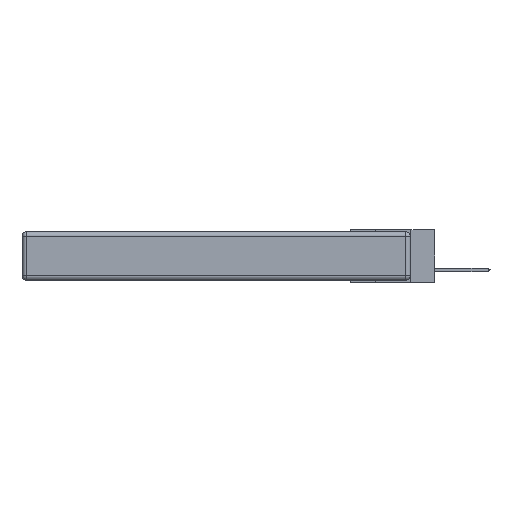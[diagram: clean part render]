
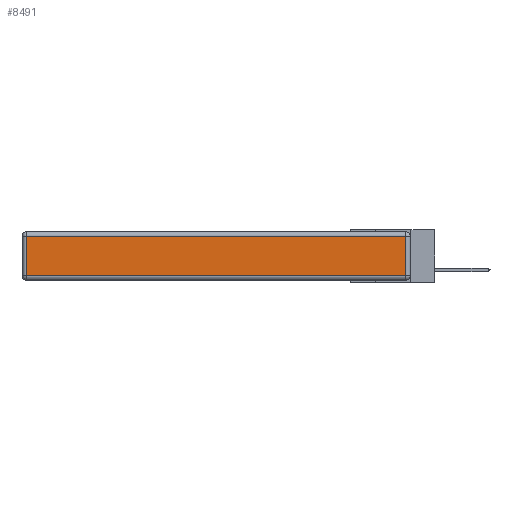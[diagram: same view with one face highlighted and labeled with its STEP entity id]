
A CAD part, left-side view. The second image highlights one B-rep face of the part: STEP entity #8491.
In plain terms, the highlighted planar face has unit normal (-1, 0, 0).
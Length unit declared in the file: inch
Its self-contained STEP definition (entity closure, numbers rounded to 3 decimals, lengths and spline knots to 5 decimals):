
#1834 = EDGE_CURVE ( 'NONE', #15540, #20115, #21368, .T. ) ;
#3686 = EDGE_CURVE ( 'NONE', #20085, #15540, #3948, .T. ) ;
#3948 = LINE ( 'NONE', #19818, #24108 ) ;
#4475 = VERTEX_POINT ( 'NONE', #6435 ) ;
#4882 = PLANE ( 'NONE',  #5160 ) ;
#5160 = AXIS2_PLACEMENT_3D ( 'NONE', #20413, #6901, #14629 ) ;
#6435 = CARTESIAN_POINT ( 'NONE',  ( 0., 2.72, -0.313 ) ) ;
#6901 = DIRECTION ( 'NONE',  ( -1., 0., 0. ) ) ;
#7764 = FACE_OUTER_BOUND ( 'NONE', #15975, .T. ) ;
#8491 = ADVANCED_FACE ( 'NONE', ( #7764 ), #4882, .T. ) ;
#8629 = LINE ( 'NONE', #18706, #10735 ) ;
#10615 = DIRECTION ( 'NONE',  ( 0., -1., 0. ) ) ;
#10735 = VECTOR ( 'NONE', #18450, 39.37008 ) ;
#10836 = ORIENTED_EDGE ( 'NONE', *, *, #1834, .T. ) ;
#10925 = EDGE_CURVE ( 'NONE', #20115, #4475, #8629, .T. ) ;
#11140 = ORIENTED_EDGE ( 'NONE', *, *, #17292, .T. ) ;
#12356 = VECTOR ( 'NONE', #18617, 39.37008 ) ;
#14629 = DIRECTION ( 'NONE',  ( 0., 0., 1. ) ) ;
#15354 = CARTESIAN_POINT ( 'NONE',  ( 0., 0.03, -0.313 ) ) ;
#15540 = VERTEX_POINT ( 'NONE', #19746 ) ;
#15975 = EDGE_LOOP ( 'NONE', ( #11140, #17421, #10836, #23685 ) ) ;
#17241 = VECTOR ( 'NONE', #10615, 39.37008 ) ;
#17292 = EDGE_CURVE ( 'NONE', #4475, #20085, #19646, .T. ) ;
#17421 = ORIENTED_EDGE ( 'NONE', *, *, #3686, .T. ) ;
#18450 = DIRECTION ( 'NONE',  ( 0., 0., -1. ) ) ;
#18617 = DIRECTION ( 'NONE',  ( 0., 1., 0. ) ) ;
#18706 = CARTESIAN_POINT ( 'NONE',  ( 0., 2.72, -0.343 ) ) ;
#19279 = CARTESIAN_POINT ( 'NONE',  ( 0., 2.72, -0.03 ) ) ;
#19646 = LINE ( 'NONE', #20233, #17241 ) ;
#19746 = CARTESIAN_POINT ( 'NONE',  ( 0., 0.03, -0.03 ) ) ;
#19818 = CARTESIAN_POINT ( 'NONE',  ( 0., 0.03, -0.343 ) ) ;
#20085 = VERTEX_POINT ( 'NONE', #15354 ) ;
#20115 = VERTEX_POINT ( 'NONE', #19279 ) ;
#20233 = CARTESIAN_POINT ( 'NONE',  ( 0., 0., -0.313 ) ) ;
#20413 = CARTESIAN_POINT ( 'NONE',  ( 0., 0., -0.343 ) ) ;
#21368 = LINE ( 'NONE', #24602, #12356 ) ;
#23623 = DIRECTION ( 'NONE',  ( 0., 0., 1. ) ) ;
#23685 = ORIENTED_EDGE ( 'NONE', *, *, #10925, .T. ) ;
#24108 = VECTOR ( 'NONE', #23623, 39.37008 ) ;
#24602 = CARTESIAN_POINT ( 'NONE',  ( 0., 2.75, -0.03 ) ) ;
